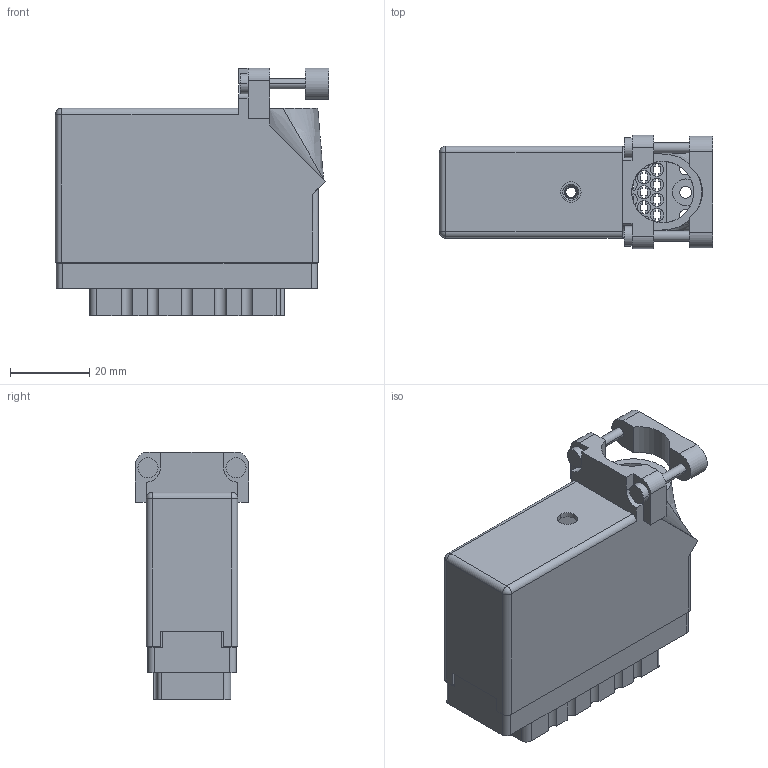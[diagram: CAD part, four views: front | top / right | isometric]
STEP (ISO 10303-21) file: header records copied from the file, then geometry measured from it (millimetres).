
FILE_DESCRIPTION (( 'STEP AP203' ), '1' );
FILE_NAME ('516-056-000-636.STEP', '2020-03-05T20:45:14', ( '' ), ( '' ), 'SwSTEP 2.0', 'SolidWorks 2016', '' );
FILE_SCHEMA (( 'CONFIG_CONTROL_DESIGN' ));
Length unit declared in the file: inch
Products named in the file (4): 516 Part Receptacle_056; 516-230-001_Plastic - 056 Top Entry - Large Clamp; 516-056-000-636; 516-252-035-100_516-252-035-100
Assembly tree (3 placements, depth 2):
  516-056-000-636
    516 Part Receptacle_056
    516-230-001_Plastic - 056 Top Entry - Large Clamp
    516-252-035-100_516-252-035-100
Bounding box: 68.91 x 28.57 x 62.51 mm (x, y, z)
Volume: 27253.6 mm3; surface area: 37503.5 mm2
Topology: 3 solids, 3 shells, 1400 faces, 4096 edges, 2724 vertices
Faces by surface type: plane 949, cylinder 428, cone 12, bspline 9, sphere 2
Entity records: 49491 total; most frequent: CARTESIAN_POINT 10763, ORIENTED_EDGE 8188, DIRECTION 7901, EDGE_CURVE 4094, VECTOR 2973, LINE 2973, VERTEX_POINT 2724, AXIS2_PLACEMENT_3D 2464
